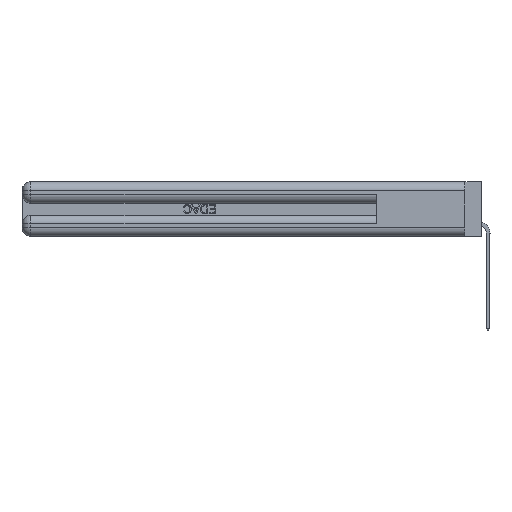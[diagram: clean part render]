
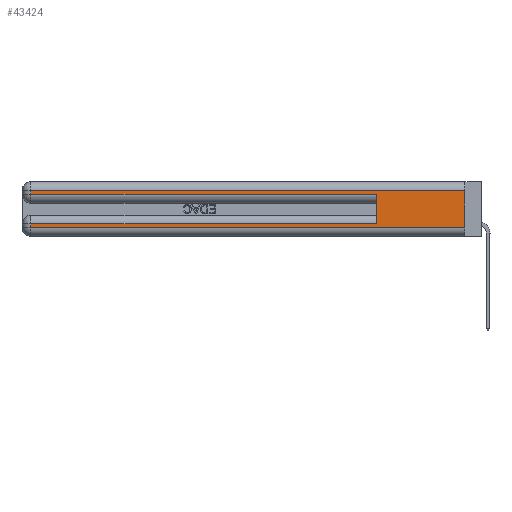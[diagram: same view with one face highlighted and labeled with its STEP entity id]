
A CAD part, left-side view. The second image highlights one B-rep face of the part: STEP entity #43424.
In plain terms, the highlighted planar face has unit normal (-1, 0, 0).
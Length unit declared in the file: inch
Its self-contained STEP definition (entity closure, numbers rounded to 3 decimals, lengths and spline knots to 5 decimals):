
#1218 = LINE ( 'NONE', #12473, #4779 ) ;
#1702 = DIRECTION ( 'NONE',  ( 0., 0., -1. ) ) ;
#3007 = EDGE_CURVE ( 'NONE', #47842, #22370, #45511, .T. ) ;
#3536 = VECTOR ( 'NONE', #1702, 39.37008 ) ;
#3792 = LINE ( 'NONE', #17459, #42152 ) ;
#4779 = VECTOR ( 'NONE', #27758, 39.37008 ) ;
#8357 = CARTESIAN_POINT ( 'NONE',  ( 0., 0.6, 0.145 ) ) ;
#8713 = CARTESIAN_POINT ( 'NONE',  ( 0., 0.6, 0.085 ) ) ;
#9175 = LINE ( 'NONE', #14003, #21916 ) ;
#9512 = CARTESIAN_POINT ( 'NONE',  ( 0., 0., 0.31 ) ) ;
#10475 = DIRECTION ( 'NONE',  ( 0., 0., -1. ) ) ;
#11388 = DIRECTION ( 'NONE',  ( 0., 1., 0. ) ) ;
#11390 = CARTESIAN_POINT ( 'NONE',  ( 0., 0., 0.06 ) ) ;
#12284 = VERTEX_POINT ( 'NONE', #24455 ) ;
#12332 = VERTEX_POINT ( 'NONE', #31762 ) ;
#12473 = CARTESIAN_POINT ( 'NONE',  ( 0., 0., 0.085 ) ) ;
#12996 = AXIS2_PLACEMENT_3D ( 'NONE', #19075, #26377, #15019 ) ;
#13370 = LINE ( 'NONE', #23806, #3536 ) ;
#13687 = CARTESIAN_POINT ( 'NONE',  ( 0., 0., 0.285 ) ) ;
#14003 = CARTESIAN_POINT ( 'NONE',  ( 0., 2.94, 0.37 ) ) ;
#14967 = DIRECTION ( 'NONE',  ( 0., -1., 0. ) ) ;
#15019 = DIRECTION ( 'NONE',  ( 0., 0., -1. ) ) ;
#15420 = VERTEX_POINT ( 'NONE', #20865 ) ;
#15644 = ORIENTED_EDGE ( 'NONE', *, *, #3007, .F. ) ;
#15819 = EDGE_CURVE ( 'NONE', #47842, #42153, #1218, .T. ) ;
#17459 = CARTESIAN_POINT ( 'NONE',  ( 0., 0., 0.31 ) ) ;
#19075 = CARTESIAN_POINT ( 'NONE',  ( 0., 0., 0.37 ) ) ;
#19259 = ORIENTED_EDGE ( 'NONE', *, *, #43106, .F. ) ;
#19350 = CARTESIAN_POINT ( 'NONE',  ( 0., 2.94, 0.085 ) ) ;
#19639 = CARTESIAN_POINT ( 'NONE',  ( 0., 0.6, 0.285 ) ) ;
#20171 = ORIENTED_EDGE ( 'NONE', *, *, #47954, .T. ) ;
#20216 = EDGE_CURVE ( 'NONE', #41768, #35689, #3792, .T. ) ;
#20865 = CARTESIAN_POINT ( 'NONE',  ( 0., 2.94, 0.06 ) ) ;
#21154 = VECTOR ( 'NONE', #38071, 39.37008 ) ;
#21916 = VECTOR ( 'NONE', #10475, 39.37008 ) ;
#21922 = ORIENTED_EDGE ( 'NONE', *, *, #29777, .T. ) ;
#22370 = VERTEX_POINT ( 'NONE', #19639 ) ;
#23806 = CARTESIAN_POINT ( 'NONE',  ( 0., 0., 0.37 ) ) ;
#24455 = CARTESIAN_POINT ( 'NONE',  ( 0., 0., 0.06 ) ) ;
#24793 = LINE ( 'NONE', #47002, #41661 ) ;
#26377 = DIRECTION ( 'NONE',  ( 1., 0., 0. ) ) ;
#26996 = ORIENTED_EDGE ( 'NONE', *, *, #15819, .T. ) ;
#27758 = DIRECTION ( 'NONE',  ( 0., 1., 0. ) ) ;
#27905 = FACE_OUTER_BOUND ( 'NONE', #39496, .T. ) ;
#28497 = ORIENTED_EDGE ( 'NONE', *, *, #38196, .T. ) ;
#29777 = EDGE_CURVE ( 'NONE', #12332, #22370, #36699, .T. ) ;
#29805 = LINE ( 'NONE', #11390, #31506 ) ;
#31506 = VECTOR ( 'NONE', #14967, 39.37008 ) ;
#31762 = CARTESIAN_POINT ( 'NONE',  ( 0., 2.94, 0.285 ) ) ;
#32266 = EDGE_CURVE ( 'NONE', #42153, #15420, #9175, .T. ) ;
#32762 = ORIENTED_EDGE ( 'NONE', *, *, #20216, .T. ) ;
#35620 = DIRECTION ( 'NONE',  ( 0., 0., -1. ) ) ;
#35689 = VERTEX_POINT ( 'NONE', #43683 ) ;
#36699 = LINE ( 'NONE', #13687, #47166 ) ;
#38071 = DIRECTION ( 'NONE',  ( 0., 0., 1. ) ) ;
#38196 = EDGE_CURVE ( 'NONE', #15420, #12284, #29805, .T. ) ;
#39496 = EDGE_LOOP ( 'NONE', ( #19259, #32762, #20171, #21922, #15644, #26996, #46450, #28497 ) ) ;
#41661 = VECTOR ( 'NONE', #35620, 39.37008 ) ;
#41768 = VERTEX_POINT ( 'NONE', #9512 ) ;
#42152 = VECTOR ( 'NONE', #11388, 39.37008 ) ;
#42153 = VERTEX_POINT ( 'NONE', #19350 ) ;
#43106 = EDGE_CURVE ( 'NONE', #41768, #12284, #13370, .T. ) ;
#43424 = ADVANCED_FACE ( 'NONE', ( #27905 ), #44452, .F. ) ;
#43683 = CARTESIAN_POINT ( 'NONE',  ( 0., 2.94, 0.31 ) ) ;
#44452 = PLANE ( 'NONE',  #12996 ) ;
#45511 = LINE ( 'NONE', #8357, #21154 ) ;
#46450 = ORIENTED_EDGE ( 'NONE', *, *, #32266, .T. ) ;
#46838 = DIRECTION ( 'NONE',  ( 0., -1., 0. ) ) ;
#47002 = CARTESIAN_POINT ( 'NONE',  ( 0., 2.94, 0.37 ) ) ;
#47166 = VECTOR ( 'NONE', #46838, 39.37008 ) ;
#47842 = VERTEX_POINT ( 'NONE', #8713 ) ;
#47954 = EDGE_CURVE ( 'NONE', #35689, #12332, #24793, .T. ) ;
